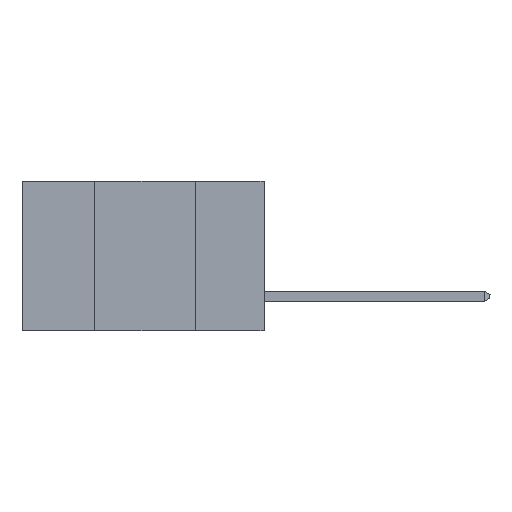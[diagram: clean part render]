
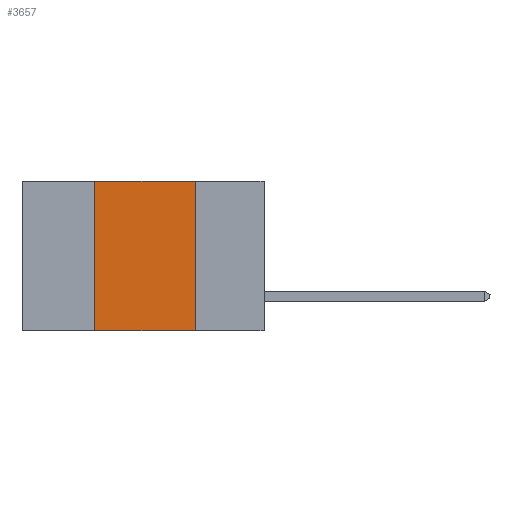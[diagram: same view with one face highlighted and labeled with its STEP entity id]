
A CAD part, left-side view. The second image highlights one B-rep face of the part: STEP entity #3657.
In plain terms, the highlighted planar face has unit normal (-1, 0, 0).
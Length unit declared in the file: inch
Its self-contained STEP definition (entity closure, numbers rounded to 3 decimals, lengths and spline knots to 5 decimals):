
#348 = VECTOR ( 'NONE', #9268, 39.37008 ) ;
#1060 = CARTESIAN_POINT ( 'NONE',  ( 0., 0.17, 0. ) ) ;
#1960 = CARTESIAN_POINT ( 'NONE',  ( 0., 0.6, -0.37 ) ) ;
#1962 = CARTESIAN_POINT ( 'NONE',  ( 0., 0.6, 0. ) ) ;
#2121 = ORIENTED_EDGE ( 'NONE', *, *, #12699, .F. ) ;
#2448 = VERTEX_POINT ( 'NONE', #9040 ) ;
#3624 = VECTOR ( 'NONE', #4174, 39.37008 ) ;
#3657 = ADVANCED_FACE ( 'NONE', ( #3839 ), #10535, .F. ) ;
#3839 = FACE_OUTER_BOUND ( 'NONE', #12876, .T. ) ;
#4174 = DIRECTION ( 'NONE',  ( 0., -1., 0. ) ) ;
#4839 = CARTESIAN_POINT ( 'NONE',  ( 0., 0.6, 0. ) ) ;
#5338 = EDGE_CURVE ( 'NONE', #2448, #10169, #12297, .T. ) ;
#5429 = ORIENTED_EDGE ( 'NONE', *, *, #5338, .T. ) ;
#5864 = CARTESIAN_POINT ( 'NONE',  ( 0., 0.17, 0. ) ) ;
#6262 = LINE ( 'NONE', #4839, #11378 ) ;
#6762 = ORIENTED_EDGE ( 'NONE', *, *, #9821, .F. ) ;
#7287 = LINE ( 'NONE', #5864, #14101 ) ;
#7551 = ORIENTED_EDGE ( 'NONE', *, *, #9302, .F. ) ;
#7938 = AXIS2_PLACEMENT_3D ( 'NONE', #1962, #11737, #12932 ) ;
#8188 = CARTESIAN_POINT ( 'NONE',  ( 0., 0.42, 0. ) ) ;
#9040 = CARTESIAN_POINT ( 'NONE',  ( 0., 0.42, -0.37 ) ) ;
#9268 = DIRECTION ( 'NONE',  ( 0., 0., 1. ) ) ;
#9302 = EDGE_CURVE ( 'NONE', #11676, #10169, #7287, .T. ) ;
#9821 = EDGE_CURVE ( 'NONE', #10900, #11676, #6262, .T. ) ;
#10169 = VERTEX_POINT ( 'NONE', #10821 ) ;
#10535 = PLANE ( 'NONE',  #7938 ) ;
#10821 = CARTESIAN_POINT ( 'NONE',  ( 0., 0.17, -0.37 ) ) ;
#10900 = VERTEX_POINT ( 'NONE', #12506 ) ;
#11197 = DIRECTION ( 'NONE',  ( 0., 0., -1. ) ) ;
#11378 = VECTOR ( 'NONE', #13544, 39.37008 ) ;
#11471 = LINE ( 'NONE', #8188, #348 ) ;
#11676 = VERTEX_POINT ( 'NONE', #1060 ) ;
#11737 = DIRECTION ( 'NONE',  ( 1., 0., 0. ) ) ;
#12297 = LINE ( 'NONE', #1960, #3624 ) ;
#12506 = CARTESIAN_POINT ( 'NONE',  ( 0., 0.42, 0. ) ) ;
#12699 = EDGE_CURVE ( 'NONE', #2448, #10900, #11471, .T. ) ;
#12876 = EDGE_LOOP ( 'NONE', ( #7551, #6762, #2121, #5429 ) ) ;
#12932 = DIRECTION ( 'NONE',  ( 0., 0., -1. ) ) ;
#13544 = DIRECTION ( 'NONE',  ( 0., -1., 0. ) ) ;
#14101 = VECTOR ( 'NONE', #11197, 39.37008 ) ;
